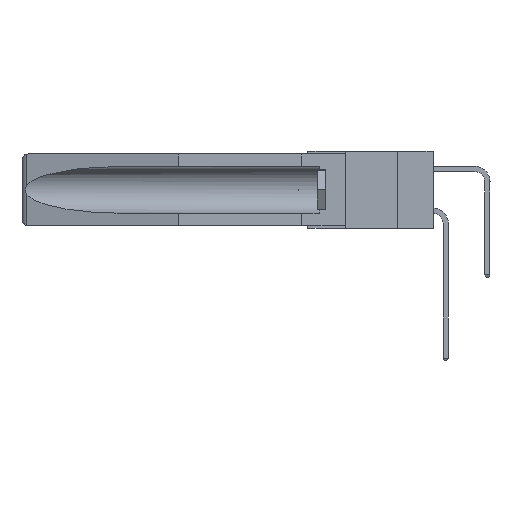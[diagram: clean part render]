
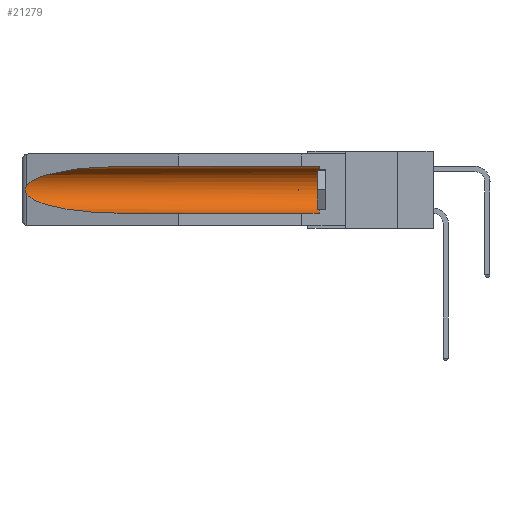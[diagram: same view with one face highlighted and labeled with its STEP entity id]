
A CAD part, left-side view. The second image highlights one B-rep face of the part: STEP entity #21279.
In plain terms, the highlighted cylindrical face has radius 2.857 mm (diameter 5.715 mm), a partial arc.
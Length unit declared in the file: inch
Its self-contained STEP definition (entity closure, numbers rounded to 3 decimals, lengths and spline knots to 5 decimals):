
#226 = CARTESIAN_POINT ( 'NONE',  ( 0.155, 1.07973, -0.284 ) ) ;
#263 = DIRECTION ( 'NONE',  ( 0., -1., 0. ) ) ;
#2347 = CARTESIAN_POINT ( 'NONE',  ( 0.26597, 1.5296, -0.19026 ) ) ;
#3846 = CARTESIAN_POINT ( 'NONE',  ( 0.155, 1.07973, -0.059 ) ) ;
#3855 =( BOUNDED_CURVE ( )  B_SPLINE_CURVE ( 3, ( #28413, #17072, #31765, #226 ),
 .UNSPECIFIED., .F., .F. ) 
 B_SPLINE_CURVE_WITH_KNOTS ( ( 4, 4 ),
 ( 0.1948, 1.5708 ),
 .UNSPECIFIED. ) 
 CURVE ( )  GEOMETRIC_REPRESENTATION_ITEM ( )  RATIONAL_B_SPLINE_CURVE ( ( 1., 0.848, 0.848, 1. ) ) 
 REPRESENTATION_ITEM ( '' )  );
#4138 = AXIS2_PLACEMENT_3D ( 'NONE', #11546, #31082, #16863 ) ;
#4748 = VERTEX_POINT ( 'NONE', #36728 ) ;
#5004 = CARTESIAN_POINT ( 'NONE',  ( 0.26537, 1.52718, -0.14972 ) ) ;
#5136 = EDGE_CURVE ( 'NONE', #4748, #23665, #13841, .T. ) ;
#5360 = CARTESIAN_POINT ( 'NONE',  ( 0.2673, 1.53269, -0.17917 ) ) ;
#5994 = ORIENTED_EDGE ( 'NONE', *, *, #32393, .T. ) ;
#8959 = LINE ( 'NONE', #20590, #28904 ) ;
#9430 = VECTOR ( 'NONE', #36020, 39.37008 ) ;
#9689 =( BOUNDED_CURVE ( )  B_SPLINE_CURVE ( 3, ( #3846, #34983, #17649, #17785 ),
 .UNSPECIFIED., .F., .F. ) 
 B_SPLINE_CURVE_WITH_KNOTS ( ( 4, 4 ),
 ( 4.71239, 6.08839 ),
 .UNSPECIFIED. ) 
 CURVE ( )  GEOMETRIC_REPRESENTATION_ITEM ( )  RATIONAL_B_SPLINE_CURVE ( ( 1., 0.848, 0.848, 1. ) ) 
 REPRESENTATION_ITEM ( '' )  );
#10323 = DIRECTION ( 'NONE',  ( 0., 1., 0. ) ) ;
#10853 = CARTESIAN_POINT ( 'NONE',  ( 0.26537, 1.52718, -0.14972 ) ) ;
#11452 = FACE_OUTER_BOUND ( 'NONE', #17956, .T. ) ;
#11546 = CARTESIAN_POINT ( 'NONE',  ( 0.155, -0.30754, -0.1715 ) ) ;
#11658 = VERTEX_POINT ( 'NONE', #5004 ) ;
#13560 = CARTESIAN_POINT ( 'NONE',  ( 0.155, -0.30754, -0.284 ) ) ;
#13677 = CARTESIAN_POINT ( 'NONE',  ( 0.26597, 1.52961, -0.15275 ) ) ;
#13837 = CIRCLE ( 'NONE', #26814, 0.1125 ) ;
#13841 = LINE ( 'NONE', #13560, #9430 ) ;
#16466 = CARTESIAN_POINT ( 'NONE',  ( 0.2675, 1.53308, -0.16763 ) ) ;
#16539 = ORIENTED_EDGE ( 'NONE', *, *, #5136, .F. ) ;
#16656 = CARTESIAN_POINT ( 'NONE',  ( 0.26655, 1.53094, -0.18657 ) ) ;
#16811 = EDGE_CURVE ( 'NONE', #22989, #22512, #8959, .T. ) ;
#16863 = DIRECTION ( 'NONE',  ( 0., 0., 1. ) ) ;
#17072 = CARTESIAN_POINT ( 'NONE',  ( 0.25451, 1.48313, -0.24835 ) ) ;
#17085 = B_SPLINE_CURVE_WITH_KNOTS ( 'NONE', 3,
 ( #10853, #13677, #34132, #19509, #16466, #27995, #5360, #16656, #2347, #31253 ),
 .UNSPECIFIED., .F., .F.,
 ( 4, 2, 2, 2, 4 ),
 ( 0., 0.00029, 0.00058, 0.00087, 0.00117 ),
 .UNSPECIFIED. ) ;
#17518 = CARTESIAN_POINT ( 'NONE',  ( 0.155, 0.126, -0.059 ) ) ;
#17587 = VERTEX_POINT ( 'NONE', #32586 ) ;
#17649 = CARTESIAN_POINT ( 'NONE',  ( 0.25451, 1.48313, -0.09465 ) ) ;
#17785 = CARTESIAN_POINT ( 'NONE',  ( 0.26537, 1.52718, -0.14972 ) ) ;
#17802 = ORIENTED_EDGE ( 'NONE', *, *, #22809, .T. ) ;
#17956 = EDGE_LOOP ( 'NONE', ( #5994, #17802, #28937, #16539, #28146, #32425 ) ) ;
#19509 = CARTESIAN_POINT ( 'NONE',  ( 0.2673, 1.5327, -0.16383 ) ) ;
#20590 = CARTESIAN_POINT ( 'NONE',  ( 0.155, -0.30754, -0.059 ) ) ;
#21279 = ADVANCED_FACE ( 'NONE', ( #11452 ), #30129, .F. ) ;
#21686 = EDGE_CURVE ( 'NONE', #17587, #23665, #3855, .T. ) ;
#22512 = VERTEX_POINT ( 'NONE', #36713 ) ;
#22515 = EDGE_CURVE ( 'NONE', #4748, #22989, #13837, .T. ) ;
#22809 = EDGE_CURVE ( 'NONE', #11658, #17587, #17085, .T. ) ;
#22989 = VERTEX_POINT ( 'NONE', #17518 ) ;
#23665 = VERTEX_POINT ( 'NONE', #33475 ) ;
#25937 = CARTESIAN_POINT ( 'NONE',  ( 0.155, 0.126, -0.1715 ) ) ;
#26814 = AXIS2_PLACEMENT_3D ( 'NONE', #25937, #263, #31700 ) ;
#27995 = CARTESIAN_POINT ( 'NONE',  ( 0.2675, 1.53308, -0.17534 ) ) ;
#28146 = ORIENTED_EDGE ( 'NONE', *, *, #22515, .T. ) ;
#28413 = CARTESIAN_POINT ( 'NONE',  ( 0.26537, 1.52718, -0.19328 ) ) ;
#28904 = VECTOR ( 'NONE', #10323, 39.37008 ) ;
#28937 = ORIENTED_EDGE ( 'NONE', *, *, #21686, .T. ) ;
#30129 = CYLINDRICAL_SURFACE ( 'NONE', #4138, 0.1125 ) ;
#31082 = DIRECTION ( 'NONE',  ( 0., 1., 0. ) ) ;
#31253 = CARTESIAN_POINT ( 'NONE',  ( 0.26537, 1.52718, -0.19328 ) ) ;
#31700 = DIRECTION ( 'NONE',  ( 0., 0., 1. ) ) ;
#31765 = CARTESIAN_POINT ( 'NONE',  ( 0.21114, 1.30732, -0.284 ) ) ;
#32393 = EDGE_CURVE ( 'NONE', #22512, #11658, #9689, .T. ) ;
#32425 = ORIENTED_EDGE ( 'NONE', *, *, #16811, .T. ) ;
#32586 = CARTESIAN_POINT ( 'NONE',  ( 0.26537, 1.52718, -0.19328 ) ) ;
#33475 = CARTESIAN_POINT ( 'NONE',  ( 0.155, 1.07973, -0.284 ) ) ;
#34132 = CARTESIAN_POINT ( 'NONE',  ( 0.26654, 1.53092, -0.15636 ) ) ;
#34983 = CARTESIAN_POINT ( 'NONE',  ( 0.21114, 1.30732, -0.059 ) ) ;
#36020 = DIRECTION ( 'NONE',  ( 0., 1., 0. ) ) ;
#36713 = CARTESIAN_POINT ( 'NONE',  ( 0.155, 1.07973, -0.059 ) ) ;
#36728 = CARTESIAN_POINT ( 'NONE',  ( 0.155, 0.126, -0.284 ) ) ;
